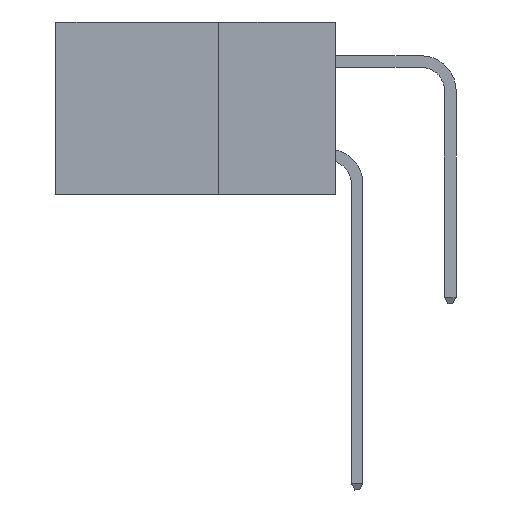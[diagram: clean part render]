
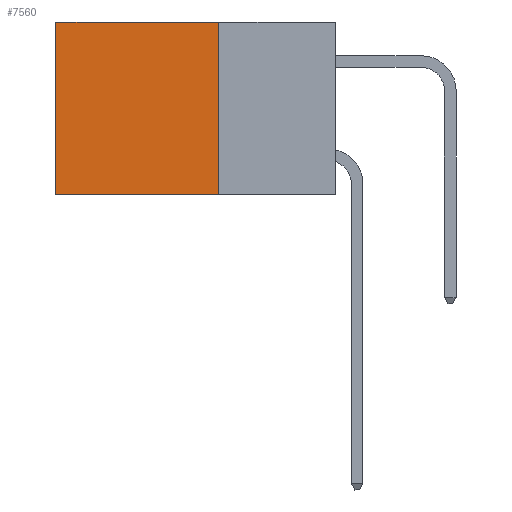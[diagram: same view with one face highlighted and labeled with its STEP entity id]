
A CAD part, left-side view. The second image highlights one B-rep face of the part: STEP entity #7560.
In plain terms, the highlighted planar face has unit normal (-1, 0, 0).
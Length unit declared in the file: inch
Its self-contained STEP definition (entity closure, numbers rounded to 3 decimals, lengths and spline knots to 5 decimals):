
#365 = CARTESIAN_POINT ( 'NONE',  ( 0.2875, 0.6, 0. ) ) ;
#2782 = LINE ( 'NONE', #365, #34486 ) ;
#3893 = CARTESIAN_POINT ( 'NONE',  ( 0.2875, 0.6, 0. ) ) ;
#4283 = AXIS2_PLACEMENT_3D ( 'NONE', #27272, #32409, #35908 ) ;
#5326 = VERTEX_POINT ( 'NONE', #5620 ) ;
#5620 = CARTESIAN_POINT ( 'NONE',  ( 0.2875, 0.25, 0. ) ) ;
#5648 = ORIENTED_EDGE ( 'NONE', *, *, #28446, .F. ) ;
#6532 = VERTEX_POINT ( 'NONE', #21102 ) ;
#6880 = VECTOR ( 'NONE', #14154, 39.37008 ) ;
#7560 = ADVANCED_FACE ( 'NONE', ( #10140 ), #21382, .F. ) ;
#9211 = CARTESIAN_POINT ( 'NONE',  ( 0.2875, 0.25, -0.37 ) ) ;
#10140 = FACE_OUTER_BOUND ( 'NONE', #32614, .T. ) ;
#11141 = CARTESIAN_POINT ( 'NONE',  ( 0.2875, 0.25, 0. ) ) ;
#11663 = VERTEX_POINT ( 'NONE', #34551 ) ;
#12085 = ORIENTED_EDGE ( 'NONE', *, *, #20444, .T. ) ;
#12713 = EDGE_CURVE ( 'NONE', #11663, #6532, #14569, .T. ) ;
#13724 = DIRECTION ( 'NONE',  ( 0., 0., -1. ) ) ;
#14030 = VERTEX_POINT ( 'NONE', #3893 ) ;
#14154 = DIRECTION ( 'NONE',  ( 0., 1., 0. ) ) ;
#14569 = LINE ( 'NONE', #9211, #29399 ) ;
#15693 = VECTOR ( 'NONE', #13724, 39.37008 ) ;
#16933 = LINE ( 'NONE', #28162, #6880 ) ;
#20376 = EDGE_CURVE ( 'NONE', #14030, #6532, #2782, .T. ) ;
#20444 = EDGE_CURVE ( 'NONE', #5326, #14030, #16933, .T. ) ;
#21102 = CARTESIAN_POINT ( 'NONE',  ( 0.2875, 0.6, -0.37 ) ) ;
#21382 = PLANE ( 'NONE',  #4283 ) ;
#23226 = DIRECTION ( 'NONE',  ( 0., 1., 0. ) ) ;
#27272 = CARTESIAN_POINT ( 'NONE',  ( 0.2875, 0.25, 0. ) ) ;
#27717 = LINE ( 'NONE', #11141, #15693 ) ;
#28162 = CARTESIAN_POINT ( 'NONE',  ( 0.2875, 0.25, 0. ) ) ;
#28446 = EDGE_CURVE ( 'NONE', #5326, #11663, #27717, .T. ) ;
#29399 = VECTOR ( 'NONE', #23226, 39.37008 ) ;
#30622 = ORIENTED_EDGE ( 'NONE', *, *, #20376, .T. ) ;
#31257 = DIRECTION ( 'NONE',  ( 0., 0., -1. ) ) ;
#31427 = ORIENTED_EDGE ( 'NONE', *, *, #12713, .F. ) ;
#32409 = DIRECTION ( 'NONE',  ( 1., 0., 0. ) ) ;
#32614 = EDGE_LOOP ( 'NONE', ( #30622, #31427, #5648, #12085 ) ) ;
#34486 = VECTOR ( 'NONE', #31257, 39.37008 ) ;
#34551 = CARTESIAN_POINT ( 'NONE',  ( 0.2875, 0.25, -0.37 ) ) ;
#35908 = DIRECTION ( 'NONE',  ( 0., 0., -1. ) ) ;
